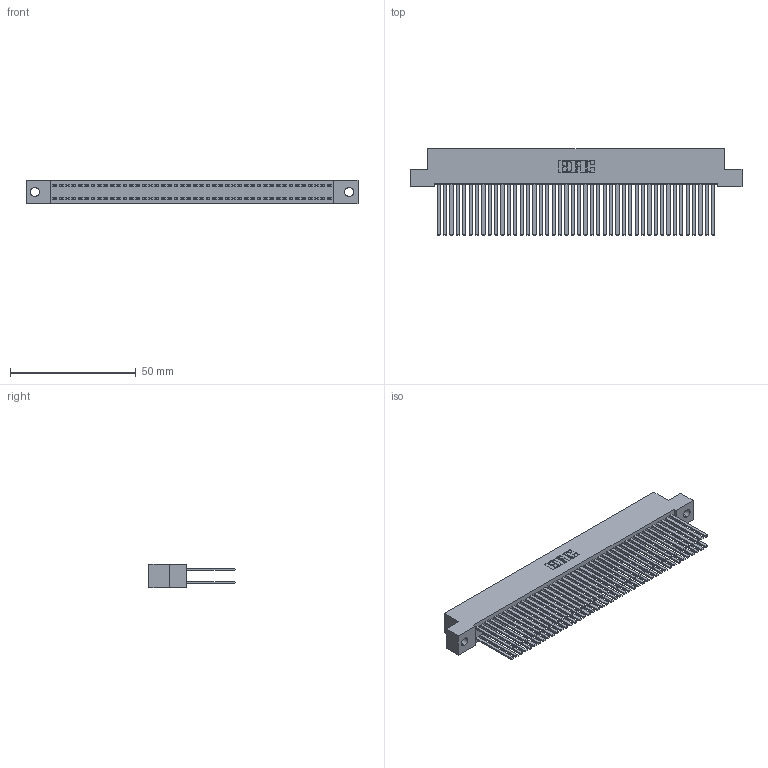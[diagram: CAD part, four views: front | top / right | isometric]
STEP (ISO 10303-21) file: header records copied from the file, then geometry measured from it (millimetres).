
FILE_DESCRIPTION (( 'STEP AP203' ), '1' );
FILE_NAME ('392-088-544-202.STEP', '2019-10-09T16:54:35', ( '' ), ( '' ), 'SwSTEP 2.0', 'SolidWorks 2016', '' );
FILE_SCHEMA (( 'CONFIG_CONTROL_DESIGN' ));
Length unit declared in the file: inch
Products named in the file (3): 345-292-001_345-293-144; 392-088-544-202; 342 Part_.128 Slot
Assembly tree (89 placements, depth 2):
  392-088-544-202
    342 Part_.128 Slot
    345-292-001_345-293-144  x88
Bounding box: 132.08 x 34.3 x 9.4 mm (x, y, z)
Volume: 13058.3 mm3; surface area: 24480.7 mm2
Topology: 89 solids, 89 shells, 4162 faces, 12367 edges, 8126 vertices
Faces by surface type: plane 2886, cylinder 1276
Entity records: 27867 total; most frequent: CARTESIAN_POINT 4614, ORIENTED_EDGE 4550, DIRECTION 3935, EDGE_CURVE 2275, VECTOR 2151, LINE 2151, VERTEX_POINT 1514, AXIS2_PLACEMENT_3D 892
